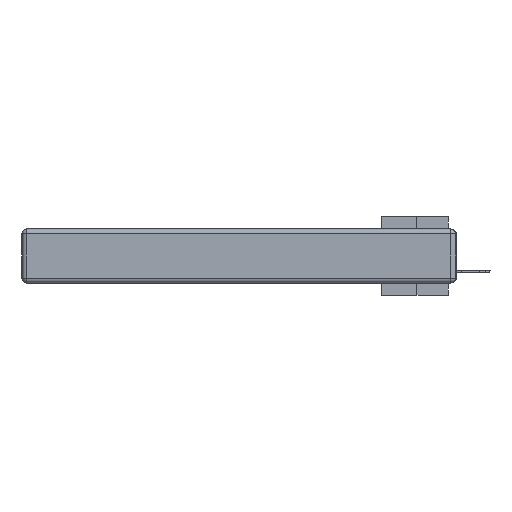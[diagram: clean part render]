
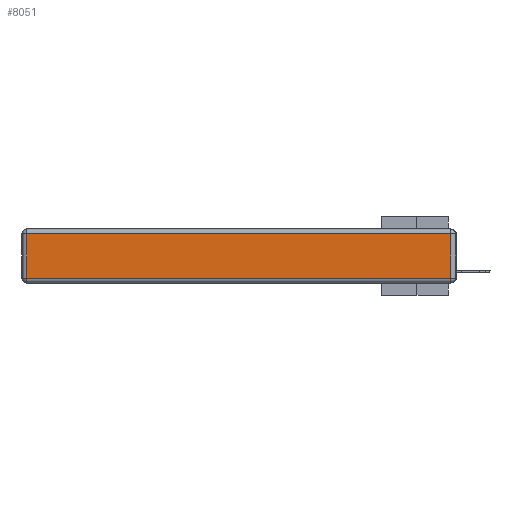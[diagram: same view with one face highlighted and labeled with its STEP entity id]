
A CAD part, left-side view. The second image highlights one B-rep face of the part: STEP entity #8051.
In plain terms, the highlighted planar face has unit normal (-1, 0, 0).
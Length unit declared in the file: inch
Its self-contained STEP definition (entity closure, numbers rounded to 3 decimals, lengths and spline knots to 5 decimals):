
#146 = CARTESIAN_POINT ( 'NONE',  ( 0., 2.72, -0.343 ) ) ;
#318 = DIRECTION ( 'NONE',  ( 0., 0., 1. ) ) ;
#2002 = CARTESIAN_POINT ( 'NONE',  ( 0., 2.72, -0.03 ) ) ;
#2777 = PLANE ( 'NONE',  #33616 ) ;
#2984 = EDGE_CURVE ( 'NONE', #23968, #31369, #5892, .T. ) ;
#4022 = EDGE_CURVE ( 'NONE', #18700, #27279, #5828, .T. ) ;
#4605 = LINE ( 'NONE', #10799, #12200 ) ;
#5828 = LINE ( 'NONE', #146, #35582 ) ;
#5892 = LINE ( 'NONE', #31988, #17192 ) ;
#6696 = CARTESIAN_POINT ( 'NONE',  ( 0., 0.03, -0.03 ) ) ;
#8051 = ADVANCED_FACE ( 'NONE', ( #8764 ), #2777, .T. ) ;
#8502 = CARTESIAN_POINT ( 'NONE',  ( 0., 0.03, -0.313 ) ) ;
#8764 = FACE_OUTER_BOUND ( 'NONE', #23363, .T. ) ;
#10799 = CARTESIAN_POINT ( 'NONE',  ( 0., 2.75, -0.03 ) ) ;
#12200 = VECTOR ( 'NONE', #36553, 39.37008 ) ;
#16051 = DIRECTION ( 'NONE',  ( 0., 0., 1. ) ) ;
#17192 = VECTOR ( 'NONE', #16051, 39.37008 ) ;
#18376 = VECTOR ( 'NONE', #24370, 39.37008 ) ;
#18596 = ORIENTED_EDGE ( 'NONE', *, *, #4022, .T. ) ;
#18700 = VERTEX_POINT ( 'NONE', #2002 ) ;
#19803 = ORIENTED_EDGE ( 'NONE', *, *, #26917, .T. ) ;
#22490 = LINE ( 'NONE', #27236, #18376 ) ;
#23363 = EDGE_LOOP ( 'NONE', ( #19803, #36844, #25714, #18596 ) ) ;
#23814 = DIRECTION ( 'NONE',  ( -1., 0., 0. ) ) ;
#23968 = VERTEX_POINT ( 'NONE', #8502 ) ;
#24370 = DIRECTION ( 'NONE',  ( 0., -1., 0. ) ) ;
#25714 = ORIENTED_EDGE ( 'NONE', *, *, #30428, .T. ) ;
#25859 = CARTESIAN_POINT ( 'NONE',  ( 0., 0., -0.343 ) ) ;
#26917 = EDGE_CURVE ( 'NONE', #27279, #23968, #22490, .T. ) ;
#27236 = CARTESIAN_POINT ( 'NONE',  ( 0., 0., -0.313 ) ) ;
#27279 = VERTEX_POINT ( 'NONE', #28131 ) ;
#28131 = CARTESIAN_POINT ( 'NONE',  ( 0., 2.72, -0.313 ) ) ;
#30428 = EDGE_CURVE ( 'NONE', #31369, #18700, #4605, .T. ) ;
#31369 = VERTEX_POINT ( 'NONE', #6696 ) ;
#31988 = CARTESIAN_POINT ( 'NONE',  ( 0., 0.03, -0.343 ) ) ;
#33616 = AXIS2_PLACEMENT_3D ( 'NONE', #25859, #23814, #318 ) ;
#34817 = DIRECTION ( 'NONE',  ( 0., 0., -1. ) ) ;
#35582 = VECTOR ( 'NONE', #34817, 39.37008 ) ;
#36553 = DIRECTION ( 'NONE',  ( 0., 1., 0. ) ) ;
#36844 = ORIENTED_EDGE ( 'NONE', *, *, #2984, .T. ) ;
